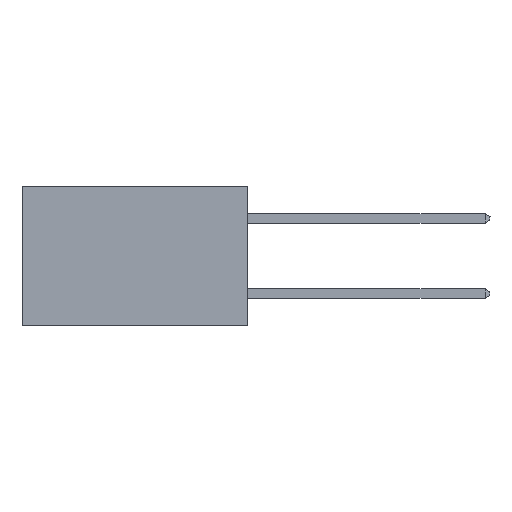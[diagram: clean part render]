
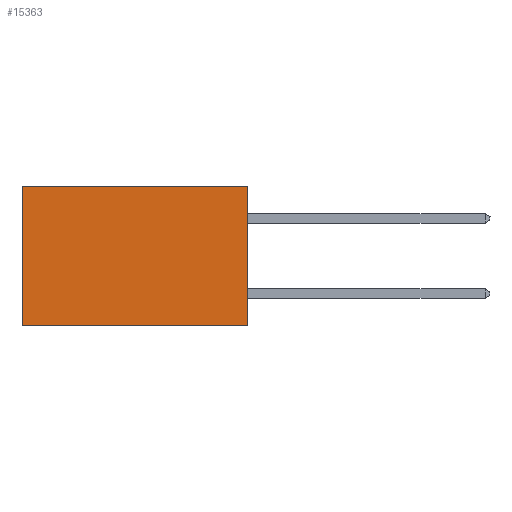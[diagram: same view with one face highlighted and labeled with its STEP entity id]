
A CAD part, left-side view. The second image highlights one B-rep face of the part: STEP entity #15363.
In plain terms, the highlighted planar face has unit normal (-1, 0, 0).
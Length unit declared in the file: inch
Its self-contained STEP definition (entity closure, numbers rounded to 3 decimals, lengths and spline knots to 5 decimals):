
#891 = VECTOR ( 'NONE', #12853, 39.37008 ) ;
#1572 = LINE ( 'NONE', #13413, #15033 ) ;
#2303 = VERTEX_POINT ( 'NONE', #16880 ) ;
#2622 = DIRECTION ( 'NONE',  ( 1., 0., 0. ) ) ;
#3380 = ORIENTED_EDGE ( 'NONE', *, *, #12630, .T. ) ;
#3702 = CARTESIAN_POINT ( 'NONE',  ( 0.2615, 0.6, 0. ) ) ;
#3981 = CARTESIAN_POINT ( 'NONE',  ( 0.2615, 0., -0.37 ) ) ;
#4520 = ORIENTED_EDGE ( 'NONE', *, *, #13707, .F. ) ;
#5375 = CARTESIAN_POINT ( 'NONE',  ( 0.2615, 0., -0.37 ) ) ;
#6004 = CARTESIAN_POINT ( 'NONE',  ( 0.2615, 0., -0.37 ) ) ;
#6283 = DIRECTION ( 'NONE',  ( 0., 0., -1. ) ) ;
#7081 = LINE ( 'NONE', #11236, #891 ) ;
#7208 = ORIENTED_EDGE ( 'NONE', *, *, #17656, .F. ) ;
#7461 = LINE ( 'NONE', #6004, #14738 ) ;
#8088 = LINE ( 'NONE', #5375, #10040 ) ;
#8551 = VERTEX_POINT ( 'NONE', #3702 ) ;
#9950 = DIRECTION ( 'NONE',  ( 0., 0., -1. ) ) ;
#10040 = VECTOR ( 'NONE', #18221, 39.37008 ) ;
#10480 = ORIENTED_EDGE ( 'NONE', *, *, #13561, .T. ) ;
#11146 = CARTESIAN_POINT ( 'NONE',  ( 0.2615, 0.6, -0.37 ) ) ;
#11236 = CARTESIAN_POINT ( 'NONE',  ( 0.2615, 0., 0. ) ) ;
#11733 = EDGE_LOOP ( 'NONE', ( #3380, #7208, #4520, #10480 ) ) ;
#12630 = EDGE_CURVE ( 'NONE', #8551, #13662, #1572, .T. ) ;
#12853 = DIRECTION ( 'NONE',  ( 0., 1., 0. ) ) ;
#12855 = VERTEX_POINT ( 'NONE', #14369 ) ;
#12881 = AXIS2_PLACEMENT_3D ( 'NONE', #3981, #2622, #9950 ) ;
#13413 = CARTESIAN_POINT ( 'NONE',  ( 0.2615, 0.6, -0.37 ) ) ;
#13561 = EDGE_CURVE ( 'NONE', #2303, #8551, #7081, .T. ) ;
#13662 = VERTEX_POINT ( 'NONE', #11146 ) ;
#13707 = EDGE_CURVE ( 'NONE', #2303, #12855, #7461, .T. ) ;
#14369 = CARTESIAN_POINT ( 'NONE',  ( 0.2615, 0., -0.37 ) ) ;
#14738 = VECTOR ( 'NONE', #17692, 39.37008 ) ;
#15033 = VECTOR ( 'NONE', #6283, 39.37008 ) ;
#15363 = ADVANCED_FACE ( 'NONE', ( #18661 ), #15761, .F. ) ;
#15761 = PLANE ( 'NONE',  #12881 ) ;
#16880 = CARTESIAN_POINT ( 'NONE',  ( 0.2615, 0., 0. ) ) ;
#17656 = EDGE_CURVE ( 'NONE', #12855, #13662, #8088, .T. ) ;
#17692 = DIRECTION ( 'NONE',  ( 0., 0., -1. ) ) ;
#18221 = DIRECTION ( 'NONE',  ( 0., 1., 0. ) ) ;
#18661 = FACE_OUTER_BOUND ( 'NONE', #11733, .T. ) ;
